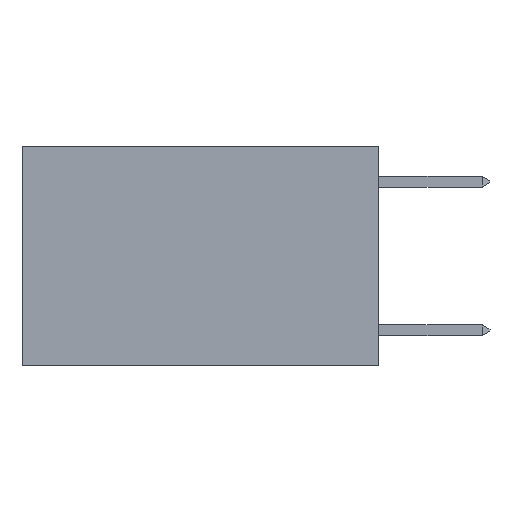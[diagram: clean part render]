
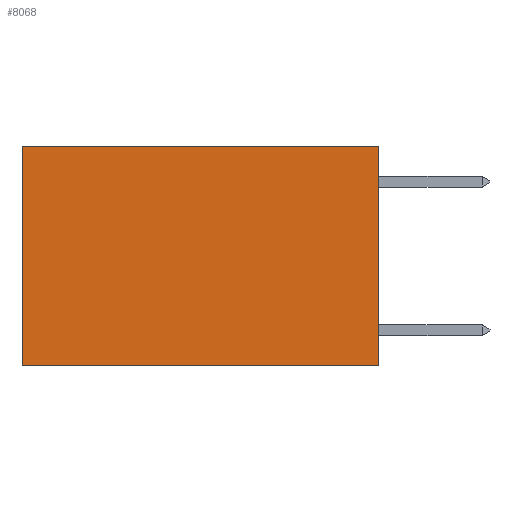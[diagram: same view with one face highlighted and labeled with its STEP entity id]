
A CAD part, left-side view. The second image highlights one B-rep face of the part: STEP entity #8068.
In plain terms, the highlighted planar face has unit normal (-1, 0, 0).
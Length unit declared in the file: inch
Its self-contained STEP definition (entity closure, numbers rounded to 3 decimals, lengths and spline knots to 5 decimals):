
#113 = CARTESIAN_POINT ( 'NONE',  ( 0.2625, 0., 0. ) ) ;
#373 = ORIENTED_EDGE ( 'NONE', *, *, #940, .F. ) ;
#504 = VECTOR ( 'NONE', #557, 39.37008 ) ;
#557 = DIRECTION ( 'NONE',  ( 0., 1., 0. ) ) ;
#575 = VECTOR ( 'NONE', #950, 39.37008 ) ;
#940 = EDGE_CURVE ( 'NONE', #4583, #9422, #6979, .T. ) ;
#950 = DIRECTION ( 'NONE',  ( 0., 0., -1. ) ) ;
#1217 = VERTEX_POINT ( 'NONE', #9352 ) ;
#1274 = CARTESIAN_POINT ( 'NONE',  ( 0.2625, 0.6, 0. ) ) ;
#2065 = ORIENTED_EDGE ( 'NONE', *, *, #8632, .F. ) ;
#2263 = CARTESIAN_POINT ( 'NONE',  ( 0.2625, 0., 0. ) ) ;
#2289 = EDGE_CURVE ( 'NONE', #6333, #1217, #6610, .T. ) ;
#2925 = AXIS2_PLACEMENT_3D ( 'NONE', #2263, #7562, #3054 ) ;
#2977 = CARTESIAN_POINT ( 'NONE',  ( 0.2625, 0.6, 0. ) ) ;
#3054 = DIRECTION ( 'NONE',  ( 0., 0., -1. ) ) ;
#3402 = VECTOR ( 'NONE', #9799, 39.37008 ) ;
#3428 = CARTESIAN_POINT ( 'NONE',  ( 0.2625, 0., -0.37 ) ) ;
#3821 = PLANE ( 'NONE',  #2925 ) ;
#4115 = FACE_OUTER_BOUND ( 'NONE', #7644, .T. ) ;
#4583 = VERTEX_POINT ( 'NONE', #113 ) ;
#5430 = LINE ( 'NONE', #6750, #3402 ) ;
#5770 = EDGE_CURVE ( 'NONE', #4583, #6333, #8955, .T. ) ;
#6000 = CARTESIAN_POINT ( 'NONE',  ( 0.2625, 0., 0. ) ) ;
#6333 = VERTEX_POINT ( 'NONE', #2977 ) ;
#6571 = ORIENTED_EDGE ( 'NONE', *, *, #5770, .T. ) ;
#6610 = LINE ( 'NONE', #1274, #575 ) ;
#6750 = CARTESIAN_POINT ( 'NONE',  ( 0.2625, 0., -0.37 ) ) ;
#6979 = LINE ( 'NONE', #7967, #8773 ) ;
#7401 = DIRECTION ( 'NONE',  ( 0., 0., -1. ) ) ;
#7562 = DIRECTION ( 'NONE',  ( 1., 0., 0. ) ) ;
#7644 = EDGE_LOOP ( 'NONE', ( #9888, #2065, #373, #6571 ) ) ;
#7967 = CARTESIAN_POINT ( 'NONE',  ( 0.2625, 0., 0. ) ) ;
#8068 = ADVANCED_FACE ( 'NONE', ( #4115 ), #3821, .F. ) ;
#8632 = EDGE_CURVE ( 'NONE', #9422, #1217, #5430, .T. ) ;
#8773 = VECTOR ( 'NONE', #7401, 39.37008 ) ;
#8955 = LINE ( 'NONE', #6000, #504 ) ;
#9352 = CARTESIAN_POINT ( 'NONE',  ( 0.2625, 0.6, -0.37 ) ) ;
#9422 = VERTEX_POINT ( 'NONE', #3428 ) ;
#9799 = DIRECTION ( 'NONE',  ( 0., 1., 0. ) ) ;
#9888 = ORIENTED_EDGE ( 'NONE', *, *, #2289, .T. ) ;
